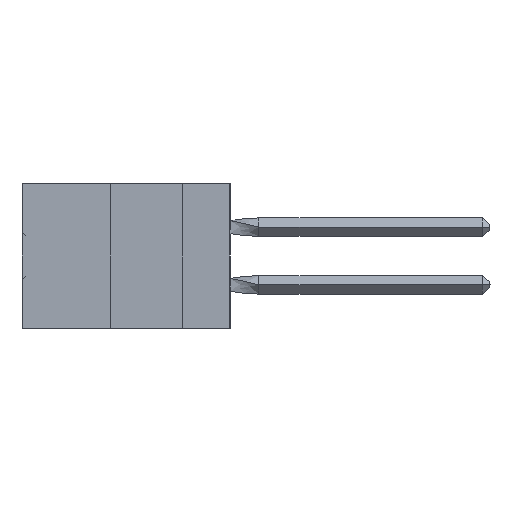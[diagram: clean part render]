
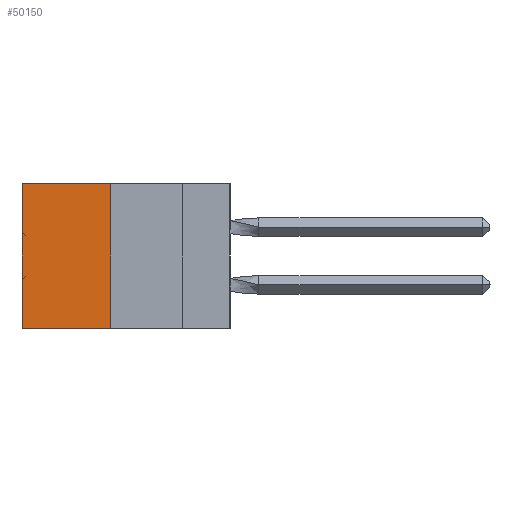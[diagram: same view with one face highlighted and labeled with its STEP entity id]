
A CAD part, left-side view. The second image highlights one B-rep face of the part: STEP entity #50150.
In plain terms, the highlighted planar face has unit normal (-1, 0, 0).
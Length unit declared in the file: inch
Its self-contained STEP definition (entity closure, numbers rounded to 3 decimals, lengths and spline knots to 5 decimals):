
#1698 = DIRECTION ( 'NONE',  ( 0., 0., -1. ) ) ;
#5284 = CARTESIAN_POINT ( 'NONE',  ( 0.305, 0.413, 0. ) ) ;
#5655 = CARTESIAN_POINT ( 'NONE',  ( 0.305, 0.413, -0.5 ) ) ;
#6972 = DIRECTION ( 'NONE',  ( 0., 1., 0. ) ) ;
#7694 = LINE ( 'NONE', #60328, #56978 ) ;
#10494 = DIRECTION ( 'NONE',  ( 0., 0., -1. ) ) ;
#11070 = VERTEX_POINT ( 'NONE', #13762 ) ;
#13762 = CARTESIAN_POINT ( 'NONE',  ( 0.305, 0.72, -0.5 ) ) ;
#17120 = VERTEX_POINT ( 'NONE', #5284 ) ;
#19085 = EDGE_CURVE ( 'NONE', #17120, #60103, #40854, .T. ) ;
#20505 = VERTEX_POINT ( 'NONE', #23249 ) ;
#21136 = CARTESIAN_POINT ( 'NONE',  ( 0.305, 0.413, -0.5 ) ) ;
#22247 = LINE ( 'NONE', #39529, #34912 ) ;
#23249 = CARTESIAN_POINT ( 'NONE',  ( 0.305, 0.413, -0.5 ) ) ;
#24824 = EDGE_LOOP ( 'NONE', ( #26437, #38544, #55515, #40848 ) ) ;
#25670 = VECTOR ( 'NONE', #58674, 39.37008 ) ;
#26437 = ORIENTED_EDGE ( 'NONE', *, *, #58160, .T. ) ;
#30983 = CARTESIAN_POINT ( 'NONE',  ( 0.305, 0.413, 0. ) ) ;
#34912 = VECTOR ( 'NONE', #1698, 39.37008 ) ;
#35988 = FACE_OUTER_BOUND ( 'NONE', #24824, .T. ) ;
#38544 = ORIENTED_EDGE ( 'NONE', *, *, #51765, .F. ) ;
#39090 = DIRECTION ( 'NONE',  ( 1., 0., 0. ) ) ;
#39529 = CARTESIAN_POINT ( 'NONE',  ( 0.305, 0.72, -0.5 ) ) ;
#40848 = ORIENTED_EDGE ( 'NONE', *, *, #19085, .T. ) ;
#40854 = LINE ( 'NONE', #30983, #49059 ) ;
#45367 = CARTESIAN_POINT ( 'NONE',  ( 0.305, 0.72, 0. ) ) ;
#49059 = VECTOR ( 'NONE', #6972, 39.37008 ) ;
#50150 = ADVANCED_FACE ( 'NONE', ( #35988 ), #58673, .F. ) ;
#51637 = AXIS2_PLACEMENT_3D ( 'NONE', #5655, #39090, #10494 ) ;
#51765 = EDGE_CURVE ( 'NONE', #20505, #11070, #54782, .T. ) ;
#54782 = LINE ( 'NONE', #21136, #25670 ) ;
#55515 = ORIENTED_EDGE ( 'NONE', *, *, #60262, .F. ) ;
#55938 = DIRECTION ( 'NONE',  ( 0., 0., -1. ) ) ;
#56978 = VECTOR ( 'NONE', #55938, 39.37008 ) ;
#58160 = EDGE_CURVE ( 'NONE', #60103, #11070, #22247, .T. ) ;
#58673 = PLANE ( 'NONE',  #51637 ) ;
#58674 = DIRECTION ( 'NONE',  ( 0., 1., 0. ) ) ;
#60103 = VERTEX_POINT ( 'NONE', #45367 ) ;
#60262 = EDGE_CURVE ( 'NONE', #17120, #20505, #7694, .T. ) ;
#60328 = CARTESIAN_POINT ( 'NONE',  ( 0.305, 0.413, -0.5 ) ) ;
